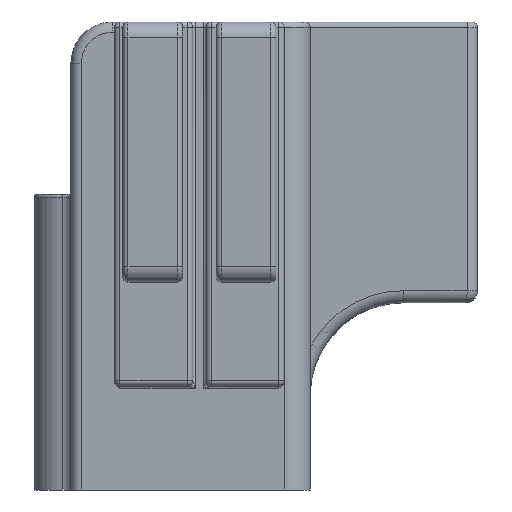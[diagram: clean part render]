
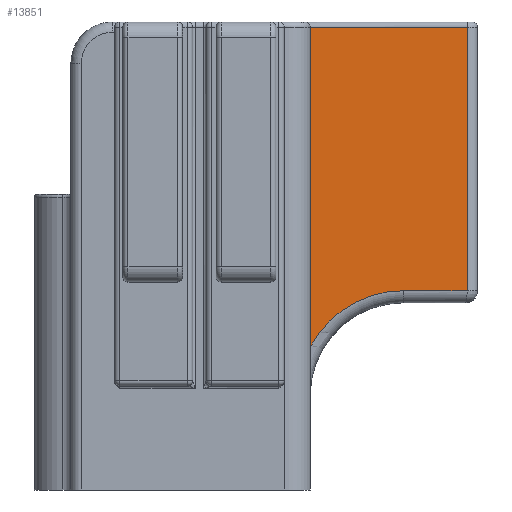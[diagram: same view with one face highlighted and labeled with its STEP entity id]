
A CAD part, front view. The second image highlights one B-rep face of the part: STEP entity #13851.
In plain terms, the highlighted planar face has unit normal (0, -1, 0).
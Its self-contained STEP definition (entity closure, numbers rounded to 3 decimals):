
#1553=PLANE('',#14583);
#2321=FACE_OUTER_BOUND('',#3105,.T.);
#3105=EDGE_LOOP('',(#12907,#12908,#12909,#12910,#12911));
#3504=CIRCLE('',#14510,20.317);
#3760=LINE('',#21037,#4588);
#3850=LINE('',#21629,#4678);
#4333=LINE('',#27952,#5161);
#4334=LINE('',#27954,#5162);
#4588=VECTOR('',#15606,10.);
#4678=VECTOR('',#16160,10.);
#5161=VECTOR('',#16837,10.);
#5162=VECTOR('',#16840,10.);
#5944=VERTEX_POINT('',#20956);
#5953=VERTEX_POINT('',#21028);
#6068=VERTEX_POINT('',#21623);
#6069=VERTEX_POINT('',#21628);
#6073=VERTEX_POINT('',#21734);
#7490=EDGE_CURVE('',#5953,#5944,#3760,.T.);
#7716=EDGE_CURVE('',#6068,#6069,#3850,.T.);
#7734=EDGE_CURVE('',#6073,#6068,#3504,.T.);
#8663=EDGE_CURVE('',#6069,#5953,#4333,.T.);
#8664=EDGE_CURVE('',#5944,#6073,#4334,.T.);
#12907=ORIENTED_EDGE('',*,*,#8663,.F.);
#12908=ORIENTED_EDGE('',*,*,#7716,.F.);
#12909=ORIENTED_EDGE('',*,*,#7734,.F.);
#12910=ORIENTED_EDGE('',*,*,#8664,.F.);
#12911=ORIENTED_EDGE('',*,*,#7490,.F.);
#13851=ADVANCED_FACE('',(#2321),#1553,.T.);
#14510=AXIS2_PLACEMENT_3D('',#21736,#16213,#16214);
#14583=AXIS2_PLACEMENT_3D('',#27953,#16838,#16839);
#15606=DIRECTION('',(0.,0.,-1.));
#16160=DIRECTION('',(0.,0.,1.));
#16213=DIRECTION('center_axis',(0.,-1.,0.));
#16214=DIRECTION('ref_axis',(-0.707,0.,0.707));
#16837=DIRECTION('',(1.,0.,0.));
#16838=DIRECTION('center_axis',(0.,-1.,0.));
#16839=DIRECTION('ref_axis',(-1.,0.,0.));
#16840=DIRECTION('',(-1.,0.,0.));
#20956=CARTESIAN_POINT('',(70.2,5.7,38.329));
#21028=CARTESIAN_POINT('',(70.2,5.7,89.));
#21037=CARTESIAN_POINT('',(70.2,5.7,90.));
#21623=CARTESIAN_POINT('',(40.,5.7,27.457));
#21628=CARTESIAN_POINT('',(40.,5.7,89.));
#21629=CARTESIAN_POINT('',(40.,5.7,45.));
#21734=CARTESIAN_POINT('',(57.988,5.7,38.329));
#21736=CARTESIAN_POINT('Origin',(57.988,5.7,18.012));
#27952=CARTESIAN_POINT('',(64.467,5.7,89.));
#27953=CARTESIAN_POINT('Origin',(67.,5.7,90.));
#27954=CARTESIAN_POINT('',(60.75,5.7,38.329));
